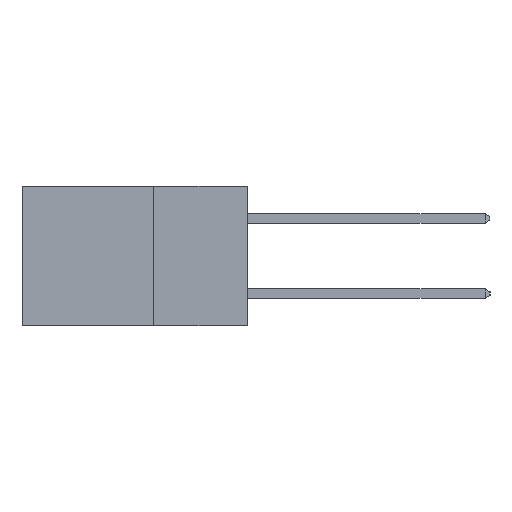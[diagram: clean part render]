
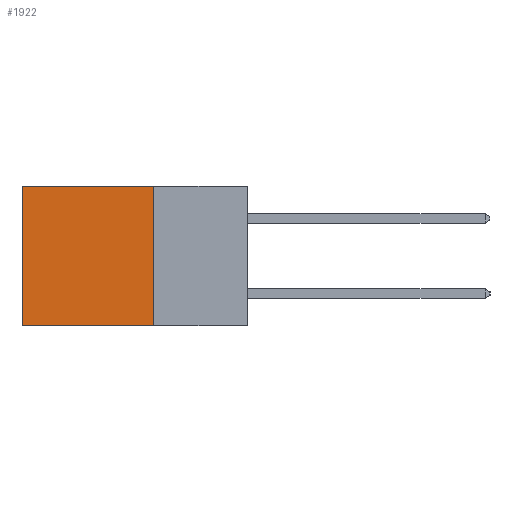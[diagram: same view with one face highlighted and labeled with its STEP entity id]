
A CAD part, left-side view. The second image highlights one B-rep face of the part: STEP entity #1922.
In plain terms, the highlighted planar face has unit normal (-1, 0, 0).
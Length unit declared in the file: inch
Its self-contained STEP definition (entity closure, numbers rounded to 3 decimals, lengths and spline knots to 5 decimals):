
#386 = VECTOR ( 'NONE', #1679, 39.37008 ) ;
#441 = VERTEX_POINT ( 'NONE', #1437 ) ;
#650 = DIRECTION ( 'NONE',  ( 0., 1., 0. ) ) ;
#799 = VERTEX_POINT ( 'NONE', #7934 ) ;
#944 = AXIS2_PLACEMENT_3D ( 'NONE', #4578, #5529, #12032 ) ;
#1437 = CARTESIAN_POINT ( 'NONE',  ( 0.2615, 0.25, -0.37 ) ) ;
#1679 = DIRECTION ( 'NONE',  ( 0., 1., 0. ) ) ;
#1850 = EDGE_CURVE ( 'NONE', #9104, #799, #8502, .T. ) ;
#1922 = ADVANCED_FACE ( 'NONE', ( #7078 ), #3628, .F. ) ;
#2549 = DIRECTION ( 'NONE',  ( 0., 0., -1. ) ) ;
#2561 = EDGE_CURVE ( 'NONE', #5757, #9104, #2739, .T. ) ;
#2656 = EDGE_CURVE ( 'NONE', #5757, #441, #4987, .T. ) ;
#2739 = LINE ( 'NONE', #7405, #386 ) ;
#2804 = ORIENTED_EDGE ( 'NONE', *, *, #2656, .F. ) ;
#3116 = ORIENTED_EDGE ( 'NONE', *, *, #2561, .T. ) ;
#3398 = VECTOR ( 'NONE', #650, 39.37008 ) ;
#3628 = PLANE ( 'NONE',  #944 ) ;
#4116 = VECTOR ( 'NONE', #11210, 39.37008 ) ;
#4539 = CARTESIAN_POINT ( 'NONE',  ( 0.2615, 0.6, 0. ) ) ;
#4578 = CARTESIAN_POINT ( 'NONE',  ( 0.2615, 0.25, -0.37 ) ) ;
#4754 = ORIENTED_EDGE ( 'NONE', *, *, #6278, .F. ) ;
#4987 = LINE ( 'NONE', #12128, #4116 ) ;
#5457 = VECTOR ( 'NONE', #2549, 39.37008 ) ;
#5529 = DIRECTION ( 'NONE',  ( 1., 0., 0. ) ) ;
#5532 = CARTESIAN_POINT ( 'NONE',  ( 0.2615, 0.25, 0. ) ) ;
#5757 = VERTEX_POINT ( 'NONE', #5532 ) ;
#5944 = LINE ( 'NONE', #12027, #3398 ) ;
#6278 = EDGE_CURVE ( 'NONE', #441, #799, #5944, .T. ) ;
#7078 = FACE_OUTER_BOUND ( 'NONE', #11238, .T. ) ;
#7299 = CARTESIAN_POINT ( 'NONE',  ( 0.2615, 0.6, -0.37 ) ) ;
#7405 = CARTESIAN_POINT ( 'NONE',  ( 0.2615, 0.25, 0. ) ) ;
#7934 = CARTESIAN_POINT ( 'NONE',  ( 0.2615, 0.6, -0.37 ) ) ;
#8502 = LINE ( 'NONE', #7299, #5457 ) ;
#9104 = VERTEX_POINT ( 'NONE', #4539 ) ;
#9395 = ORIENTED_EDGE ( 'NONE', *, *, #1850, .T. ) ;
#11210 = DIRECTION ( 'NONE',  ( 0., 0., -1. ) ) ;
#11238 = EDGE_LOOP ( 'NONE', ( #9395, #4754, #2804, #3116 ) ) ;
#12027 = CARTESIAN_POINT ( 'NONE',  ( 0.2615, 0.25, -0.37 ) ) ;
#12032 = DIRECTION ( 'NONE',  ( 0., 0., -1. ) ) ;
#12128 = CARTESIAN_POINT ( 'NONE',  ( 0.2615, 0.25, -0.37 ) ) ;
